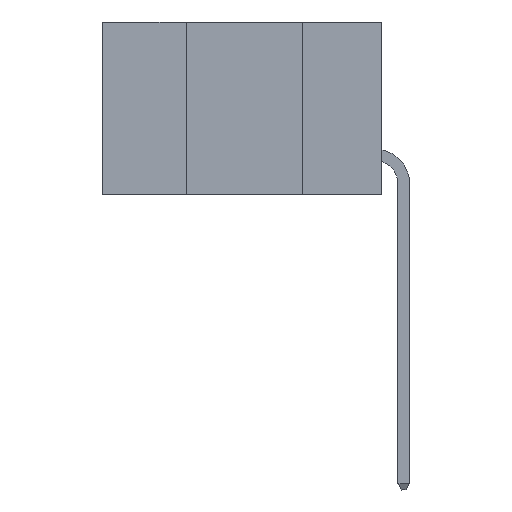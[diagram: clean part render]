
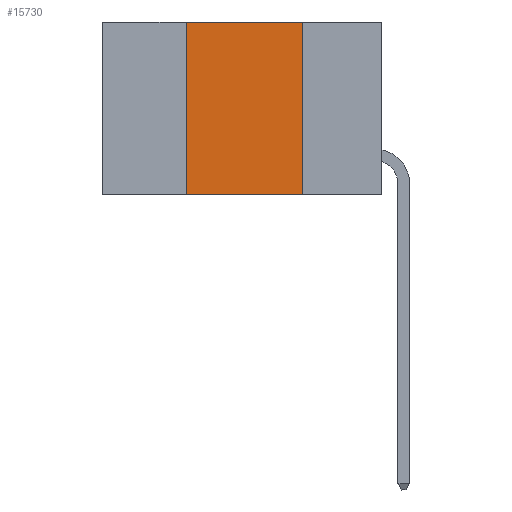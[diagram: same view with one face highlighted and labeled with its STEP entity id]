
A CAD part, left-side view. The second image highlights one B-rep face of the part: STEP entity #15730.
In plain terms, the highlighted planar face has unit normal (-1, 0, 0).
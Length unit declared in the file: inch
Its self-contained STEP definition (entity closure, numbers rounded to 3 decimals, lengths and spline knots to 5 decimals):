
#399 = EDGE_CURVE ( 'NONE', #13756, #9503, #14459, .T. ) ;
#869 = ORIENTED_EDGE ( 'NONE', *, *, #3797, .F. ) ;
#913 = LINE ( 'NONE', #2827, #8634 ) ;
#1105 = FACE_OUTER_BOUND ( 'NONE', #13293, .T. ) ;
#2549 = DIRECTION ( 'NONE',  ( 0., 0., -1. ) ) ;
#2827 = CARTESIAN_POINT ( 'NONE',  ( 0., 0.17, 0. ) ) ;
#3797 = EDGE_CURVE ( 'NONE', #9510, #12686, #13021, .T. ) ;
#4919 = CARTESIAN_POINT ( 'NONE',  ( 0., 0.6, -0.37 ) ) ;
#5024 = CARTESIAN_POINT ( 'NONE',  ( 0., 0.17, -0.37 ) ) ;
#5921 = ORIENTED_EDGE ( 'NONE', *, *, #399, .T. ) ;
#6372 = ORIENTED_EDGE ( 'NONE', *, *, #7644, .F. ) ;
#7360 = CARTESIAN_POINT ( 'NONE',  ( 0., 0.6, 0. ) ) ;
#7644 = EDGE_CURVE ( 'NONE', #13756, #9510, #9207, .T. ) ;
#8285 = PLANE ( 'NONE',  #9571 ) ;
#8435 = DIRECTION ( 'NONE',  ( 0., 0., 1. ) ) ;
#8634 = VECTOR ( 'NONE', #12957, 39.37008 ) ;
#8752 = VECTOR ( 'NONE', #8435, 39.37008 ) ;
#9141 = VECTOR ( 'NONE', #15991, 39.37008 ) ;
#9207 = LINE ( 'NONE', #12762, #8752 ) ;
#9452 = CARTESIAN_POINT ( 'NONE',  ( 0., 0.17, 0. ) ) ;
#9503 = VERTEX_POINT ( 'NONE', #5024 ) ;
#9510 = VERTEX_POINT ( 'NONE', #13725 ) ;
#9571 = AXIS2_PLACEMENT_3D ( 'NONE', #18345, #11182, #2549 ) ;
#11182 = DIRECTION ( 'NONE',  ( 1., 0., 0. ) ) ;
#12686 = VERTEX_POINT ( 'NONE', #9452 ) ;
#12762 = CARTESIAN_POINT ( 'NONE',  ( 0., 0.42, 0. ) ) ;
#12957 = DIRECTION ( 'NONE',  ( 0., 0., -1. ) ) ;
#13021 = LINE ( 'NONE', #7360, #9141 ) ;
#13293 = EDGE_LOOP ( 'NONE', ( #16242, #869, #6372, #5921 ) ) ;
#13314 = CARTESIAN_POINT ( 'NONE',  ( 0., 0.42, -0.37 ) ) ;
#13725 = CARTESIAN_POINT ( 'NONE',  ( 0., 0.42, 0. ) ) ;
#13756 = VERTEX_POINT ( 'NONE', #13314 ) ;
#14025 = VECTOR ( 'NONE', #17907, 39.37008 ) ;
#14459 = LINE ( 'NONE', #4919, #14025 ) ;
#14766 = EDGE_CURVE ( 'NONE', #12686, #9503, #913, .T. ) ;
#15730 = ADVANCED_FACE ( 'NONE', ( #1105 ), #8285, .F. ) ;
#15991 = DIRECTION ( 'NONE',  ( 0., -1., 0. ) ) ;
#16242 = ORIENTED_EDGE ( 'NONE', *, *, #14766, .F. ) ;
#17907 = DIRECTION ( 'NONE',  ( 0., -1., 0. ) ) ;
#18345 = CARTESIAN_POINT ( 'NONE',  ( 0., 0.6, 0. ) ) ;
